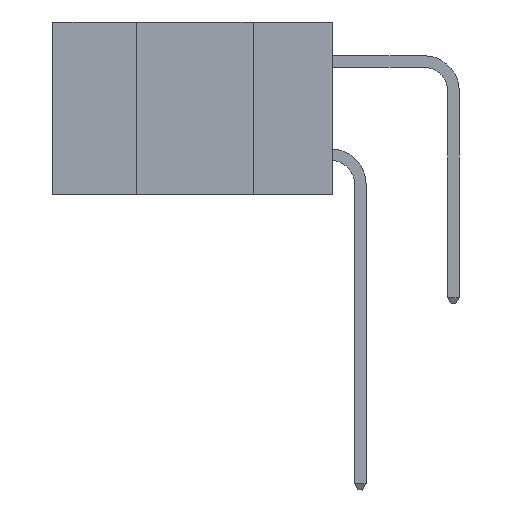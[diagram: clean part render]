
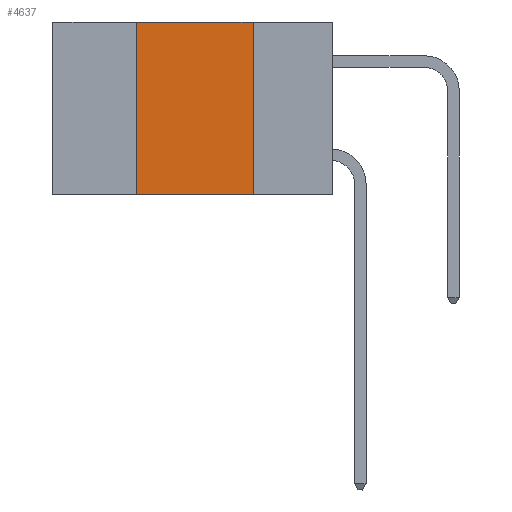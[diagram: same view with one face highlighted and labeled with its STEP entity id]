
A CAD part, left-side view. The second image highlights one B-rep face of the part: STEP entity #4637.
In plain terms, the highlighted planar face has unit normal (-1, 0, 0).
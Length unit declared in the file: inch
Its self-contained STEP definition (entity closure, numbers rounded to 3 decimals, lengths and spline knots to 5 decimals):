
#470 = CARTESIAN_POINT ( 'NONE',  ( 0., 0.6, 0. ) ) ;
#619 = AXIS2_PLACEMENT_3D ( 'NONE', #470, #7382, #6571 ) ;
#750 = VECTOR ( 'NONE', #6608, 39.37008 ) ;
#981 = VECTOR ( 'NONE', #2478, 39.37008 ) ;
#1725 = EDGE_CURVE ( 'NONE', #9365, #2593, #3454, .T. ) ;
#1767 = LINE ( 'NONE', #5294, #3232 ) ;
#2270 = CARTESIAN_POINT ( 'NONE',  ( 0., 0.42, -0.37 ) ) ;
#2478 = DIRECTION ( 'NONE',  ( 0., -1., 0. ) ) ;
#2593 = VERTEX_POINT ( 'NONE', #10382 ) ;
#2820 = ORIENTED_EDGE ( 'NONE', *, *, #3649, .F. ) ;
#3058 = ORIENTED_EDGE ( 'NONE', *, *, #1725, .T. ) ;
#3076 = LINE ( 'NONE', #2270, #750 ) ;
#3232 = VECTOR ( 'NONE', #6217, 39.37008 ) ;
#3376 = EDGE_CURVE ( 'NONE', #7372, #2593, #6811, .T. ) ;
#3454 = LINE ( 'NONE', #5361, #981 ) ;
#3649 = EDGE_CURVE ( 'NONE', #9365, #8386, #3076, .T. ) ;
#4637 = ADVANCED_FACE ( 'NONE', ( #5589 ), #9176, .F. ) ;
#5294 = CARTESIAN_POINT ( 'NONE',  ( 0., 0.6, 0. ) ) ;
#5361 = CARTESIAN_POINT ( 'NONE',  ( 0., 0.6, -0.37 ) ) ;
#5589 = FACE_OUTER_BOUND ( 'NONE', #11060, .T. ) ;
#5786 = CARTESIAN_POINT ( 'NONE',  ( 0., 0.42, -0.37 ) ) ;
#6136 = EDGE_CURVE ( 'NONE', #8386, #7372, #1767, .T. ) ;
#6217 = DIRECTION ( 'NONE',  ( 0., -1., 0. ) ) ;
#6571 = DIRECTION ( 'NONE',  ( 0., 0., -1. ) ) ;
#6608 = DIRECTION ( 'NONE',  ( 0., 0., 1. ) ) ;
#6811 = LINE ( 'NONE', #11021, #10372 ) ;
#7044 = CARTESIAN_POINT ( 'NONE',  ( 0., 0.17, 0. ) ) ;
#7372 = VERTEX_POINT ( 'NONE', #7044 ) ;
#7382 = DIRECTION ( 'NONE',  ( 1., 0., 0. ) ) ;
#7582 = ORIENTED_EDGE ( 'NONE', *, *, #3376, .F. ) ;
#8291 = ORIENTED_EDGE ( 'NONE', *, *, #6136, .F. ) ;
#8386 = VERTEX_POINT ( 'NONE', #8487 ) ;
#8487 = CARTESIAN_POINT ( 'NONE',  ( 0., 0.42, 0. ) ) ;
#9176 = PLANE ( 'NONE',  #619 ) ;
#9365 = VERTEX_POINT ( 'NONE', #5786 ) ;
#10336 = DIRECTION ( 'NONE',  ( 0., 0., -1. ) ) ;
#10372 = VECTOR ( 'NONE', #10336, 39.37008 ) ;
#10382 = CARTESIAN_POINT ( 'NONE',  ( 0., 0.17, -0.37 ) ) ;
#11021 = CARTESIAN_POINT ( 'NONE',  ( 0., 0.17, -0.37 ) ) ;
#11060 = EDGE_LOOP ( 'NONE', ( #7582, #8291, #2820, #3058 ) ) ;
